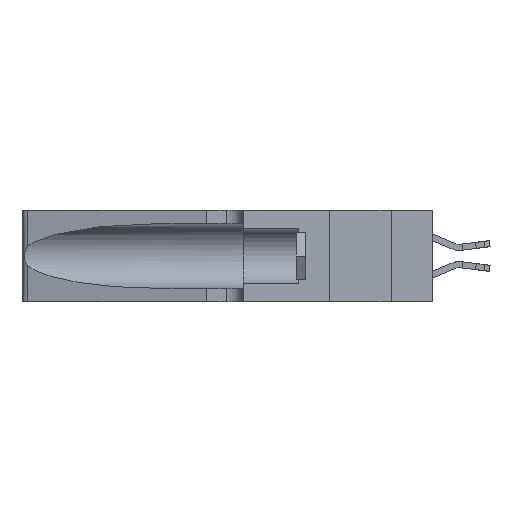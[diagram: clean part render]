
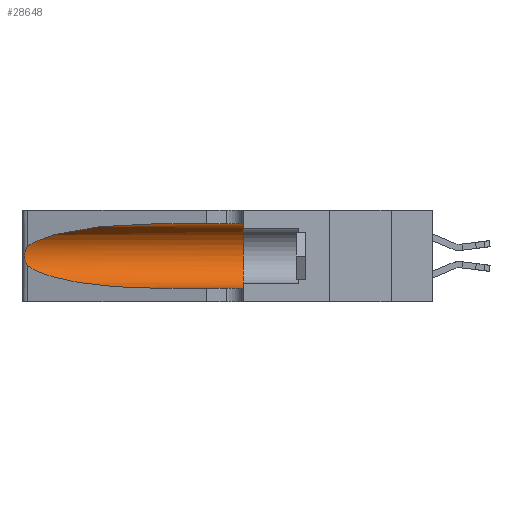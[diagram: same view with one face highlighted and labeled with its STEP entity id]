
A CAD part, left-side view. The second image highlights one B-rep face of the part: STEP entity #28648.
In plain terms, the highlighted cylindrical face has radius 3.308 mm (diameter 6.617 mm), a partial arc.
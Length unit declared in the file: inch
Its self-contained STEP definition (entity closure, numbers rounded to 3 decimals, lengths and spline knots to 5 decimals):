
#282 = VERTEX_POINT ( 'NONE', #555 ) ;
#555 = CARTESIAN_POINT ( 'NONE',  ( 0.25487, 1.22718, 0.22369 ) ) ;
#1124 = DIRECTION ( 'NONE',  ( 0., -1., 0. ) ) ;
#2006 = CARTESIAN_POINT ( 'NONE',  ( 0.1305, 1.61858, 0.31525 ) ) ;
#2539 = CARTESIAN_POINT ( 'NONE',  ( 0.26075, 1.23896, 0.178 ) ) ;
#2835 = ORIENTED_EDGE ( 'NONE', *, *, #5427, .T. ) ;
#2937 = ORIENTED_EDGE ( 'NONE', *, *, #13522, .T. ) ;
#2983 = EDGE_CURVE ( 'NONE', #23789, #9535, #12065, .T. ) ;
#3144 = VECTOR ( 'NONE', #30439, 39.37008 ) ;
#3294 = CIRCLE ( 'NONE', #9436, 0.13025 ) ;
#3920 = CARTESIAN_POINT ( 'NONE',  ( 0.25487, 1.22718, 0.22369 ) ) ;
#4519 = CARTESIAN_POINT ( 'NONE',  ( 0.25487, 1.22718, 0.14631 ) ) ;
#4770 = DIRECTION ( 'NONE',  ( 0., 1., 0. ) ) ;
#4902 = EDGE_CURVE ( 'NONE', #20002, #20818, #3294, .T. ) ;
#5390 = CARTESIAN_POINT ( 'NONE',  ( 0.25856, 1.23593, 0.16098 ) ) ;
#5427 = EDGE_CURVE ( 'NONE', #21531, #282, #15877, .T. ) ;
#7989 = CARTESIAN_POINT ( 'NONE',  ( 0.25487, 1.22718, 0.14631 ) ) ;
#8276 = CARTESIAN_POINT ( 'NONE',  ( 0.25639, 1.23186, 0.15144 ) ) ;
#9436 = AXIS2_PLACEMENT_3D ( 'NONE', #21615, #4770, #24411 ) ;
#9444 = ORIENTED_EDGE ( 'NONE', *, *, #31844, .F. ) ;
#9535 = VERTEX_POINT ( 'NONE', #27609 ) ;
#9701 = CARTESIAN_POINT ( 'NONE',  ( 0.1305, 1.61858, 0.185 ) ) ;
#9769 = ORIENTED_EDGE ( 'NONE', *, *, #4902, .F. ) ;
#10238 = CARTESIAN_POINT ( 'NONE',  ( 0.1305, 0.72297, 0.05475 ) ) ;
#10344 = CARTESIAN_POINT ( 'NONE',  ( 0.25555, 1.22994, 0.2215 ) ) ;
#10470 = CARTESIAN_POINT ( 'NONE',  ( 0.25487, 1.22718, 0.22369 ) ) ;
#11095 = CARTESIAN_POINT ( 'NONE',  ( 0.25487, 1.22718, 0.14631 ) ) ;
#11605 = EDGE_CURVE ( 'NONE', #9535, #20818, #25535, .T. ) ;
#12065 =( BOUNDED_CURVE ( )  B_SPLINE_CURVE ( 3, ( #4519, #21346, #15736, #10238 ),
 .UNSPECIFIED., .F., .F. ) 
 B_SPLINE_CURVE_WITH_KNOTS ( ( 4, 4 ),
 ( 3.44316, 4.71239 ),
 .UNSPECIFIED. ) 
 CURVE ( )  GEOMETRIC_REPRESENTATION_ITEM ( )  RATIONAL_B_SPLINE_CURVE ( ( 1., 0.87, 0.87, 1. ) ) 
 REPRESENTATION_ITEM ( '' )  );
#12491 = DIRECTION ( 'NONE',  ( 0., 0., -1. ) ) ;
#13522 = EDGE_CURVE ( 'NONE', #282, #23789, #32581, .T. ) ;
#13608 = AXIS2_PLACEMENT_3D ( 'NONE', #9701, #1124, #12491 ) ;
#13757 = CARTESIAN_POINT ( 'NONE',  ( 0.25639, 1.23184, 0.21858 ) ) ;
#15026 = VECTOR ( 'NONE', #35487, 39.37008 ) ;
#15736 = CARTESIAN_POINT ( 'NONE',  ( 0.18966, 0.96281, 0.05475 ) ) ;
#15877 =( BOUNDED_CURVE ( )  B_SPLINE_CURVE ( 3, ( #17951, #31775, #20745, #3920 ),
 .UNSPECIFIED., .F., .F. ) 
 B_SPLINE_CURVE_WITH_KNOTS ( ( 4, 4 ),
 ( 1.5708, 2.84003 ),
 .UNSPECIFIED. ) 
 CURVE ( )  GEOMETRIC_REPRESENTATION_ITEM ( )  RATIONAL_B_SPLINE_CURVE ( ( 1., 0.87, 0.87, 1. ) ) 
 REPRESENTATION_ITEM ( '' )  );
#16581 = CARTESIAN_POINT ( 'NONE',  ( 0.1305, 1.61858, 0.05475 ) ) ;
#16588 = CARTESIAN_POINT ( 'NONE',  ( 0.25854, 1.2359, 0.20912 ) ) ;
#17636 = FACE_OUTER_BOUND ( 'NONE', #29228, .T. ) ;
#17951 = CARTESIAN_POINT ( 'NONE',  ( 0.1305, 0.72297, 0.31525 ) ) ;
#18839 = ORIENTED_EDGE ( 'NONE', *, *, #2983, .T. ) ;
#19398 = CARTESIAN_POINT ( 'NONE',  ( 0.26075, 1.23896, 0.19203 ) ) ;
#20002 = VERTEX_POINT ( 'NONE', #29662 ) ;
#20477 = CARTESIAN_POINT ( 'NONE',  ( 0.1305, 0.72297, 0.31525 ) ) ;
#20745 = CARTESIAN_POINT ( 'NONE',  ( 0.2373, 1.15595, 0.28018 ) ) ;
#20818 = VERTEX_POINT ( 'NONE', #31447 ) ;
#21346 = CARTESIAN_POINT ( 'NONE',  ( 0.2373, 1.15595, 0.08982 ) ) ;
#21531 = VERTEX_POINT ( 'NONE', #20477 ) ;
#21615 = CARTESIAN_POINT ( 'NONE',  ( 0.1305, 0.35, 0.185 ) ) ;
#22218 = CARTESIAN_POINT ( 'NONE',  ( 0.26017, 1.23833, 0.17102 ) ) ;
#23503 = ORIENTED_EDGE ( 'NONE', *, *, #11605, .T. ) ;
#23789 = VERTEX_POINT ( 'NONE', #7989 ) ;
#24411 = DIRECTION ( 'NONE',  ( 0., 0., 1. ) ) ;
#25015 = CARTESIAN_POINT ( 'NONE',  ( 0.25789, 1.23486, 0.15765 ) ) ;
#25535 = LINE ( 'NONE', #16581, #3144 ) ;
#27609 = CARTESIAN_POINT ( 'NONE',  ( 0.1305, 0.72297, 0.05475 ) ) ;
#27792 = CARTESIAN_POINT ( 'NONE',  ( 0.25555, 1.22993, 0.14849 ) ) ;
#28648 = ADVANCED_FACE ( 'NONE', ( #17636 ), #31527, .F. ) ;
#29228 = EDGE_LOOP ( 'NONE', ( #2835, #2937, #18839, #23503, #9769, #9444 ) ) ;
#29662 = CARTESIAN_POINT ( 'NONE',  ( 0.1305, 0.35, 0.31525 ) ) ;
#29833 = LINE ( 'NONE', #2006, #15026 ) ;
#30439 = DIRECTION ( 'NONE',  ( 0., -1., 0. ) ) ;
#31447 = CARTESIAN_POINT ( 'NONE',  ( 0.1305, 0.35, 0.05475 ) ) ;
#31527 = CYLINDRICAL_SURFACE ( 'NONE', #13608, 0.13025 ) ;
#31775 = CARTESIAN_POINT ( 'NONE',  ( 0.18966, 0.96281, 0.31525 ) ) ;
#31844 = EDGE_CURVE ( 'NONE', #21531, #20002, #29833, .T. ) ;
#32581 = B_SPLINE_CURVE_WITH_KNOTS ( 'NONE', 3,
 ( #10470, #10344, #13757, #33239, #16588, #36011, #19398, #2539, #22218, #5390, #25015, #8276, #27792, #11095 ),
 .UNSPECIFIED., .F., .F.,
 ( 4, 2, 2, 2, 2, 2, 4 ),
 ( 0., 0.00027, 0.00053, 0.00107, 0.0016, 0.00187, 0.00214 ),
 .UNSPECIFIED. ) ;
#33239 = CARTESIAN_POINT ( 'NONE',  ( 0.25787, 1.23484, 0.2124 ) ) ;
#35487 = DIRECTION ( 'NONE',  ( 0., -1., 0. ) ) ;
#36011 = CARTESIAN_POINT ( 'NONE',  ( 0.26018, 1.23835, 0.19895 ) ) ;
